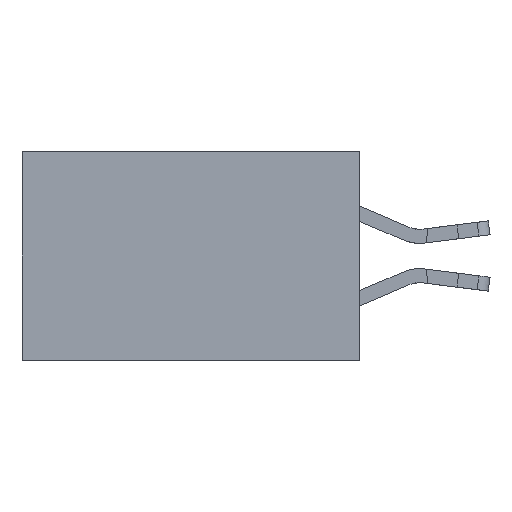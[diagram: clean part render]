
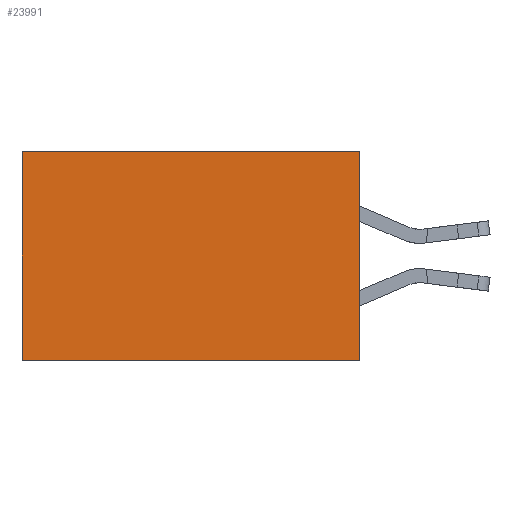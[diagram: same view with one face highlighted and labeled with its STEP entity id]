
A CAD part, left-side view. The second image highlights one B-rep face of the part: STEP entity #23991.
In plain terms, the highlighted planar face has unit normal (-1, 0, 0).
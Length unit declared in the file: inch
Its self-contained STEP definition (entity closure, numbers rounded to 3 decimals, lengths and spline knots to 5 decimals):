
#110 = EDGE_CURVE ( 'NONE', #6033, #32276, #28191, .T. ) ;
#2149 = ORIENTED_EDGE ( 'NONE', *, *, #30206, .T. ) ;
#2156 = VECTOR ( 'NONE', #2332, 39.37008 ) ;
#2169 = VERTEX_POINT ( 'NONE', #7223 ) ;
#2314 = VECTOR ( 'NONE', #30290, 39.37008 ) ;
#2332 = DIRECTION ( 'NONE',  ( 0., 1., 0. ) ) ;
#5577 = FACE_OUTER_BOUND ( 'NONE', #21576, .T. ) ;
#6033 = VERTEX_POINT ( 'NONE', #9547 ) ;
#6064 = AXIS2_PLACEMENT_3D ( 'NONE', #17988, #23065, #8116 ) ;
#6092 = DIRECTION ( 'NONE',  ( 0., 0., -1. ) ) ;
#7223 = CARTESIAN_POINT ( 'NONE',  ( 0.2875, 0.6, 0. ) ) ;
#8116 = DIRECTION ( 'NONE',  ( 0., 0., -1. ) ) ;
#8264 = ORIENTED_EDGE ( 'NONE', *, *, #8603, .T. ) ;
#8603 = EDGE_CURVE ( 'NONE', #2169, #31232, #15801, .T. ) ;
#9547 = CARTESIAN_POINT ( 'NONE',  ( 0.2875, 0., 0. ) ) ;
#10791 = ORIENTED_EDGE ( 'NONE', *, *, #20143, .F. ) ;
#11348 = LINE ( 'NONE', #32097, #14105 ) ;
#13176 = CARTESIAN_POINT ( 'NONE',  ( 0.2875, 0., 0. ) ) ;
#14105 = VECTOR ( 'NONE', #29663, 39.37008 ) ;
#15009 = VECTOR ( 'NONE', #6092, 39.37008 ) ;
#15801 = LINE ( 'NONE', #25427, #2314 ) ;
#17988 = CARTESIAN_POINT ( 'NONE',  ( 0.2875, 0., 0. ) ) ;
#18100 = PLANE ( 'NONE',  #6064 ) ;
#20143 = EDGE_CURVE ( 'NONE', #32276, #31232, #11348, .T. ) ;
#21576 = EDGE_LOOP ( 'NONE', ( #8264, #10791, #27342, #2149 ) ) ;
#21620 = CARTESIAN_POINT ( 'NONE',  ( 0.2875, 0., -0.37 ) ) ;
#23065 = DIRECTION ( 'NONE',  ( 1., 0., 0. ) ) ;
#23786 = CARTESIAN_POINT ( 'NONE',  ( 0.2875, 0.6, -0.37 ) ) ;
#23991 = ADVANCED_FACE ( 'NONE', ( #5577 ), #18100, .F. ) ;
#25427 = CARTESIAN_POINT ( 'NONE',  ( 0.2875, 0.6, 0. ) ) ;
#27342 = ORIENTED_EDGE ( 'NONE', *, *, #110, .F. ) ;
#28191 = LINE ( 'NONE', #13176, #15009 ) ;
#28815 = LINE ( 'NONE', #32254, #2156 ) ;
#29663 = DIRECTION ( 'NONE',  ( 0., 1., 0. ) ) ;
#30206 = EDGE_CURVE ( 'NONE', #6033, #2169, #28815, .T. ) ;
#30290 = DIRECTION ( 'NONE',  ( 0., 0., -1. ) ) ;
#31232 = VERTEX_POINT ( 'NONE', #23786 ) ;
#32097 = CARTESIAN_POINT ( 'NONE',  ( 0.2875, 0., -0.37 ) ) ;
#32254 = CARTESIAN_POINT ( 'NONE',  ( 0.2875, 0., 0. ) ) ;
#32276 = VERTEX_POINT ( 'NONE', #21620 ) ;
